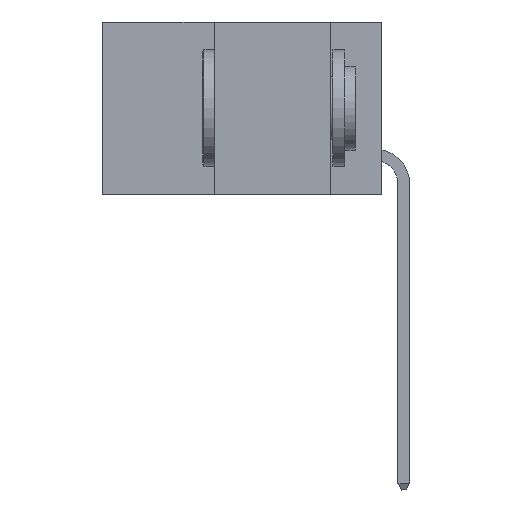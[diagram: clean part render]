
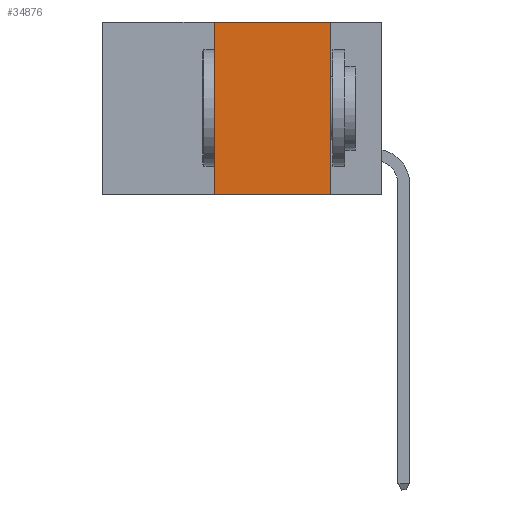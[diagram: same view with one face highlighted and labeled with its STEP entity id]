
A CAD part, left-side view. The second image highlights one B-rep face of the part: STEP entity #34876.
In plain terms, the highlighted planar face has unit normal (-1, 0, 0).
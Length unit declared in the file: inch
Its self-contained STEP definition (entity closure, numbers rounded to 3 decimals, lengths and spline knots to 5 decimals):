
#753 = EDGE_LOOP ( 'NONE', ( #20137, #18843, #19910, #10817 ) ) ;
#794 = VECTOR ( 'NONE', #37649, 39.37008 ) ;
#1515 = VECTOR ( 'NONE', #7625, 39.37008 ) ;
#3954 = VERTEX_POINT ( 'NONE', #15088 ) ;
#4956 = CARTESIAN_POINT ( 'NONE',  ( 0., 0.6, 0. ) ) ;
#4962 = VERTEX_POINT ( 'NONE', #18787 ) ;
#5006 = CARTESIAN_POINT ( 'NONE',  ( 0., 0.6, 0. ) ) ;
#5258 = PLANE ( 'NONE',  #35331 ) ;
#6291 = DIRECTION ( 'NONE',  ( 0., 0., -1. ) ) ;
#7625 = DIRECTION ( 'NONE',  ( 0., 0., 1. ) ) ;
#8043 = VECTOR ( 'NONE', #6291, 39.37008 ) ;
#9009 = CARTESIAN_POINT ( 'NONE',  ( 0., 0.11, 0. ) ) ;
#9481 = LINE ( 'NONE', #31561, #1515 ) ;
#10817 = ORIENTED_EDGE ( 'NONE', *, *, #28289, .T. ) ;
#11349 = FACE_OUTER_BOUND ( 'NONE', #753, .T. ) ;
#15088 = CARTESIAN_POINT ( 'NONE',  ( 0., 0.11, 0. ) ) ;
#16112 = CARTESIAN_POINT ( 'NONE',  ( 0., 0.6, -0.37 ) ) ;
#18787 = CARTESIAN_POINT ( 'NONE',  ( 0., 0.11, -0.37 ) ) ;
#18843 = ORIENTED_EDGE ( 'NONE', *, *, #37984, .F. ) ;
#19538 = VERTEX_POINT ( 'NONE', #23939 ) ;
#19910 = ORIENTED_EDGE ( 'NONE', *, *, #30973, .F. ) ;
#19986 = DIRECTION ( 'NONE',  ( 0., 0., -1. ) ) ;
#20137 = ORIENTED_EDGE ( 'NONE', *, *, #31306, .F. ) ;
#23849 = LINE ( 'NONE', #9009, #8043 ) ;
#23939 = CARTESIAN_POINT ( 'NONE',  ( 0., 0.36, -0.37 ) ) ;
#28289 = EDGE_CURVE ( 'NONE', #19538, #4962, #33320, .T. ) ;
#28832 = LINE ( 'NONE', #4956, #794 ) ;
#28835 = DIRECTION ( 'NONE',  ( 1., 0., 0. ) ) ;
#30049 = VECTOR ( 'NONE', #36963, 39.37008 ) ;
#30973 = EDGE_CURVE ( 'NONE', #19538, #38176, #9481, .T. ) ;
#31306 = EDGE_CURVE ( 'NONE', #3954, #4962, #23849, .T. ) ;
#31561 = CARTESIAN_POINT ( 'NONE',  ( 0., 0.36, 0. ) ) ;
#32282 = CARTESIAN_POINT ( 'NONE',  ( 0., 0.36, 0. ) ) ;
#33320 = LINE ( 'NONE', #16112, #30049 ) ;
#34876 = ADVANCED_FACE ( 'NONE', ( #11349 ), #5258, .F. ) ;
#35331 = AXIS2_PLACEMENT_3D ( 'NONE', #5006, #28835, #19986 ) ;
#36963 = DIRECTION ( 'NONE',  ( 0., -1., 0. ) ) ;
#37649 = DIRECTION ( 'NONE',  ( 0., -1., 0. ) ) ;
#37984 = EDGE_CURVE ( 'NONE', #38176, #3954, #28832, .T. ) ;
#38176 = VERTEX_POINT ( 'NONE', #32282 ) ;
